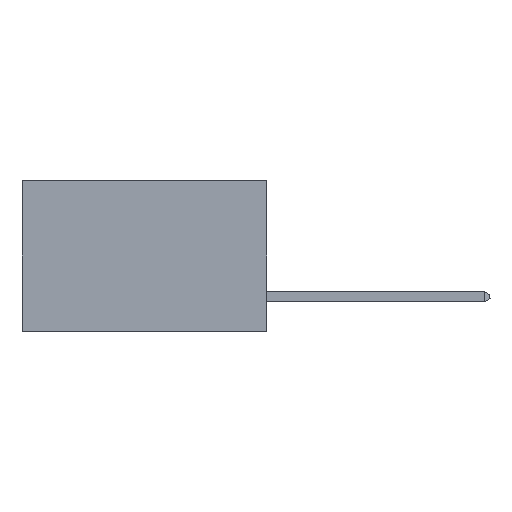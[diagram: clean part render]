
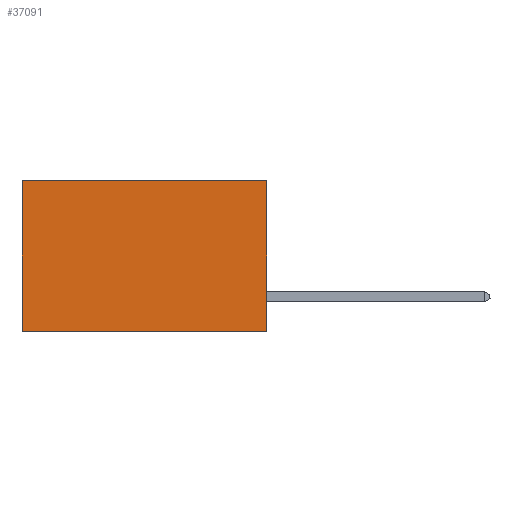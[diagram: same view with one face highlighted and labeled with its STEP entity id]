
A CAD part, left-side view. The second image highlights one B-rep face of the part: STEP entity #37091.
In plain terms, the highlighted planar face has unit normal (-1, 0, 0).
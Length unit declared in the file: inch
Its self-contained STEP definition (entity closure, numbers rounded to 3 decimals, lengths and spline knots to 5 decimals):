
#3570 = VERTEX_POINT ( 'NONE', #42469 ) ;
#6910 = DIRECTION ( 'NONE',  ( 1., 0., 0. ) ) ;
#11772 = ORIENTED_EDGE ( 'NONE', *, *, #46226, .F. ) ;
#12464 = FACE_OUTER_BOUND ( 'NONE', #35943, .T. ) ;
#14049 = CARTESIAN_POINT ( 'NONE',  ( 0.2875, 0.6, 0. ) ) ;
#17640 = VERTEX_POINT ( 'NONE', #14049 ) ;
#17745 = LINE ( 'NONE', #27649, #27237 ) ;
#17898 = CARTESIAN_POINT ( 'NONE',  ( 0.2875, 0., 0. ) ) ;
#18781 = CARTESIAN_POINT ( 'NONE',  ( 0.2875, 0., 0. ) ) ;
#19728 = CARTESIAN_POINT ( 'NONE',  ( 0.2875, 0., -0.37 ) ) ;
#20074 = EDGE_CURVE ( 'NONE', #3570, #33978, #29259, .T. ) ;
#23097 = EDGE_CURVE ( 'NONE', #3570, #17640, #24565, .T. ) ;
#23204 = CARTESIAN_POINT ( 'NONE',  ( 0.2875, 0.6, -0.37 ) ) ;
#24565 = LINE ( 'NONE', #43520, #42168 ) ;
#24975 = VECTOR ( 'NONE', #47740, 39.37008 ) ;
#25574 = ORIENTED_EDGE ( 'NONE', *, *, #32428, .T. ) ;
#27237 = VECTOR ( 'NONE', #38955, 39.37008 ) ;
#27649 = CARTESIAN_POINT ( 'NONE',  ( 0.2875, 0.6, 0. ) ) ;
#29259 = LINE ( 'NONE', #18781, #42088 ) ;
#32428 = EDGE_CURVE ( 'NONE', #17640, #35514, #17745, .T. ) ;
#33459 = AXIS2_PLACEMENT_3D ( 'NONE', #17898, #6910, #44187 ) ;
#33978 = VERTEX_POINT ( 'NONE', #19728 ) ;
#35411 = ORIENTED_EDGE ( 'NONE', *, *, #23097, .T. ) ;
#35514 = VERTEX_POINT ( 'NONE', #23204 ) ;
#35943 = EDGE_LOOP ( 'NONE', ( #25574, #11772, #46027, #35411 ) ) ;
#37091 = ADVANCED_FACE ( 'NONE', ( #12464 ), #40266, .F. ) ;
#38478 = DIRECTION ( 'NONE',  ( 0., 0., -1. ) ) ;
#38955 = DIRECTION ( 'NONE',  ( 0., 0., -1. ) ) ;
#40099 = DIRECTION ( 'NONE',  ( 0., 1., 0. ) ) ;
#40266 = PLANE ( 'NONE',  #33459 ) ;
#40281 = LINE ( 'NONE', #46926, #24975 ) ;
#42088 = VECTOR ( 'NONE', #38478, 39.37008 ) ;
#42168 = VECTOR ( 'NONE', #40099, 39.37008 ) ;
#42469 = CARTESIAN_POINT ( 'NONE',  ( 0.2875, 0., 0. ) ) ;
#43520 = CARTESIAN_POINT ( 'NONE',  ( 0.2875, 0., 0. ) ) ;
#44187 = DIRECTION ( 'NONE',  ( 0., 0., -1. ) ) ;
#46027 = ORIENTED_EDGE ( 'NONE', *, *, #20074, .F. ) ;
#46226 = EDGE_CURVE ( 'NONE', #33978, #35514, #40281, .T. ) ;
#46926 = CARTESIAN_POINT ( 'NONE',  ( 0.2875, 0., -0.37 ) ) ;
#47740 = DIRECTION ( 'NONE',  ( 0., 1., 0. ) ) ;
